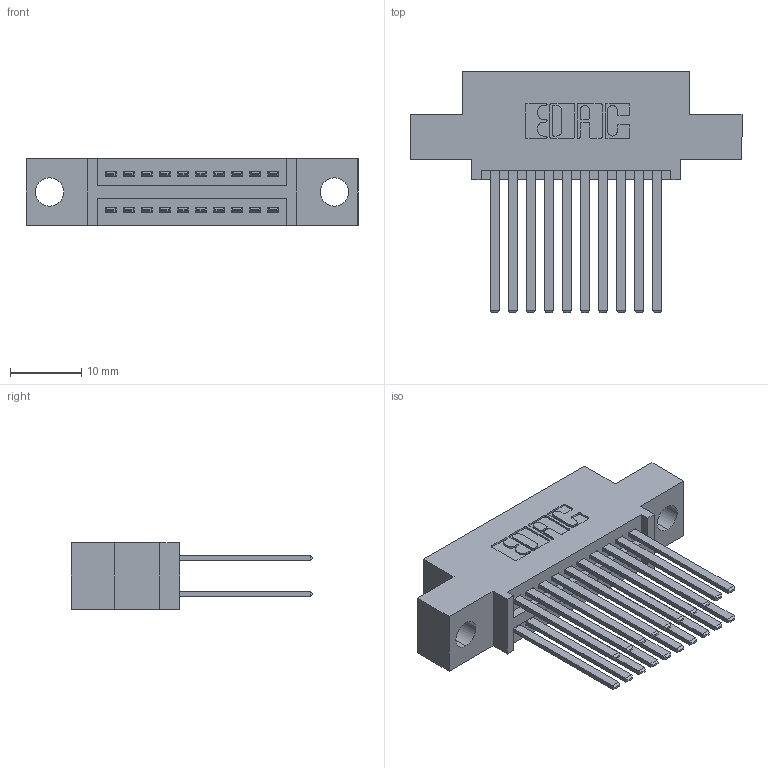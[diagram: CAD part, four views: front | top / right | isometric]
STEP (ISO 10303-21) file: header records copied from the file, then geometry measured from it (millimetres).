
FILE_DESCRIPTION (( 'STEP AP203' ), '1' );
FILE_NAME ('395-020-544-504.STEP', '2021-06-16T18:38:38', ( '' ), ( '' ), 'SwSTEP 2.0', 'SolidWorks 2020', '' );
FILE_SCHEMA (( 'CONFIG_CONTROL_DESIGN' ));
Length unit declared in the file: inch
Products named in the file (3): 345 Part_0.110 Offset - 0.156 Dia-TI; 345-292-001_345-293-144; 395-020-544-504
Assembly tree (21 placements, depth 2):
  395-020-544-504
    345 Part_0.110 Offset - 0.156 Dia-TI
    345-292-001_345-293-144  x20
Bounding box: 46.61 x 33.96 x 9.4 mm (x, y, z)
Volume: 4331.7 mm3; surface area: 6549.3 mm2
Topology: 21 solids, 21 shells, 1024 faces, 3009 edges, 1978 vertices
Faces by surface type: plane 678, cylinder 346
Entity records: 12521 total; most frequent: CARTESIAN_POINT 2134, ORIENTED_EDGE 2066, DIRECTION 1917, EDGE_CURVE 1033, LINE 865, VECTOR 865, VERTEX_POINT 686, AXIS2_PLACEMENT_3D 526
